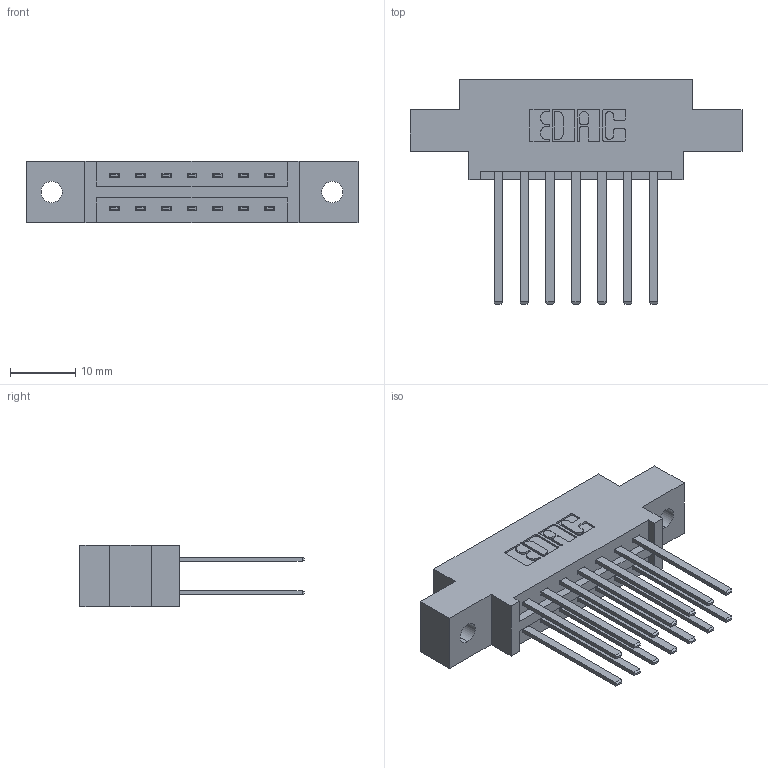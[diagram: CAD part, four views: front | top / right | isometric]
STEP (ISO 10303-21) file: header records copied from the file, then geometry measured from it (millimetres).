
FILE_DESCRIPTION (( 'STEP AP203' ), '1' );
FILE_NAME ('337-014-544-802.STEP', '2019-10-10T17:08:31', ( '' ), ( '' ), 'SwSTEP 2.0', 'SolidWorks 2016', '' );
FILE_SCHEMA (( 'CONFIG_CONTROL_DESIGN' ));
Length unit declared in the file: inch
Products named in the file (3): 345-292-001_345-293-144; 337-014-544-802; 337 Part_0.170 Offset - 0.128 Dia
Assembly tree (15 placements, depth 2):
  337-014-544-802
    337 Part_0.170 Offset - 0.128 Dia
    345-292-001_345-293-144  x14
Bounding box: 50.75 x 34.3 x 9.4 mm (x, y, z)
Volume: 4924.5 mm3; surface area: 5703.4 mm2
Topology: 15 solids, 15 shells, 790 faces, 2325 edges, 1530 vertices
Faces by surface type: plane 550, cylinder 240
Entity records: 9905 total; most frequent: CARTESIAN_POINT 1698, ORIENTED_EDGE 1634, DIRECTION 1505, EDGE_CURVE 817, VECTOR 693, LINE 693, VERTEX_POINT 542, AXIS2_PLACEMENT_3D 406
